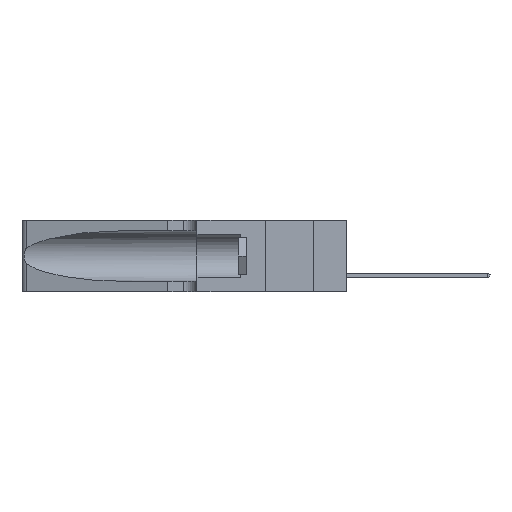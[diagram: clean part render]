
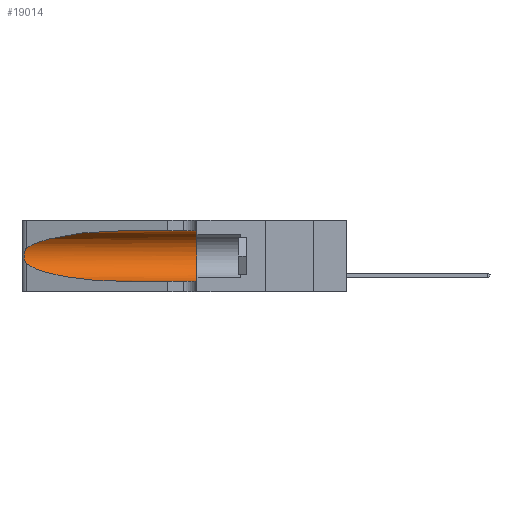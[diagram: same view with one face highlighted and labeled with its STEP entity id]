
A CAD part, left-side view. The second image highlights one B-rep face of the part: STEP entity #19014.
In plain terms, the highlighted cylindrical face has radius 3.308 mm (diameter 6.617 mm), a partial arc.
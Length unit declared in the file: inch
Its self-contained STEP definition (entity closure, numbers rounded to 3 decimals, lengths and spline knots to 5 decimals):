
#493 = VERTEX_POINT ( 'NONE', #6409 ) ;
#699 = EDGE_CURVE ( 'NONE', #23663, #19252, #7303, .T. ) ;
#864 = CARTESIAN_POINT ( 'NONE',  ( 0.1305, 0.35, 0.05475 ) ) ;
#1110 = EDGE_CURVE ( 'NONE', #493, #20791, #5302, .T. ) ;
#1565 = CARTESIAN_POINT ( 'NONE',  ( 0.26018, 1.23835, 0.19895 ) ) ;
#2272 = DIRECTION ( 'NONE',  ( 0., -1., 0. ) ) ;
#2475 = CYLINDRICAL_SURFACE ( 'NONE', #6468, 0.13025 ) ;
#3185 = DIRECTION ( 'NONE',  ( 0., 1., 0. ) ) ;
#3629 = CARTESIAN_POINT ( 'NONE',  ( 0.18966, 0.96281, 0.31525 ) ) ;
#3681 = CARTESIAN_POINT ( 'NONE',  ( 0.25856, 1.23593, 0.16098 ) ) ;
#5292 = CARTESIAN_POINT ( 'NONE',  ( 0.25487, 1.22718, 0.22369 ) ) ;
#5302 = LINE ( 'NONE', #24086, #6964 ) ;
#5741 = CARTESIAN_POINT ( 'NONE',  ( 0.25787, 1.23484, 0.2124 ) ) ;
#6034 = CARTESIAN_POINT ( 'NONE',  ( 0.2373, 1.15595, 0.28018 ) ) ;
#6409 = CARTESIAN_POINT ( 'NONE',  ( 0.1305, 0.72297, 0.05475 ) ) ;
#6468 = AXIS2_PLACEMENT_3D ( 'NONE', #24821, #9857, #7535 ) ;
#6730 = ORIENTED_EDGE ( 'NONE', *, *, #699, .F. ) ;
#6964 = VECTOR ( 'NONE', #2272, 39.37008 ) ;
#7047 = ORIENTED_EDGE ( 'NONE', *, *, #1110, .T. ) ;
#7303 = LINE ( 'NONE', #17247, #10281 ) ;
#7535 = DIRECTION ( 'NONE',  ( 0., 0., -1. ) ) ;
#7867 = CARTESIAN_POINT ( 'NONE',  ( 0.25639, 1.23186, 0.15144 ) ) ;
#8730 = DIRECTION ( 'NONE',  ( 0., -1., 0. ) ) ;
#9497 = CARTESIAN_POINT ( 'NONE',  ( 0.1305, 0.35, 0.185 ) ) ;
#9857 = DIRECTION ( 'NONE',  ( 0., -1., 0. ) ) ;
#10097 = FACE_OUTER_BOUND ( 'NONE', #18028, .T. ) ;
#10281 = VECTOR ( 'NONE', #8730, 39.37008 ) ;
#11514 = DIRECTION ( 'NONE',  ( 0., 0., 1. ) ) ;
#11858 = CARTESIAN_POINT ( 'NONE',  ( 0.25639, 1.23184, 0.21858 ) ) ;
#12005 = CARTESIAN_POINT ( 'NONE',  ( 0.1305, 0.72297, 0.05475 ) ) ;
#12075 = AXIS2_PLACEMENT_3D ( 'NONE', #9497, #3185, #11514 ) ;
#12823 = B_SPLINE_CURVE_WITH_KNOTS ( 'NONE', 3,
 ( #18354, #22823, #11858, #5741, #24591, #1565, #16399, #20304, #26755, #3681, #20674, #7867, #16484, #24966 ),
 .UNSPECIFIED., .F., .F.,
 ( 4, 2, 2, 2, 2, 2, 4 ),
 ( 0., 0.00027, 0.00053, 0.00107, 0.0016, 0.00187, 0.00214 ),
 .UNSPECIFIED. ) ;
#13263 = ORIENTED_EDGE ( 'NONE', *, *, #19708, .T. ) ;
#13898 = CARTESIAN_POINT ( 'NONE',  ( 0.25487, 1.22718, 0.14631 ) ) ;
#14076 = CARTESIAN_POINT ( 'NONE',  ( 0.18966, 0.96281, 0.05475 ) ) ;
#14173 = CARTESIAN_POINT ( 'NONE',  ( 0.25487, 1.22718, 0.14631 ) ) ;
#14568 = EDGE_CURVE ( 'NONE', #23663, #24562, #19451, .T. ) ;
#15636 = EDGE_CURVE ( 'NONE', #24767, #493, #25606, .T. ) ;
#15726 = ORIENTED_EDGE ( 'NONE', *, *, #15636, .T. ) ;
#16330 = CARTESIAN_POINT ( 'NONE',  ( 0.1305, 0.72297, 0.31525 ) ) ;
#16399 = CARTESIAN_POINT ( 'NONE',  ( 0.26075, 1.23896, 0.19203 ) ) ;
#16484 = CARTESIAN_POINT ( 'NONE',  ( 0.25555, 1.22993, 0.14849 ) ) ;
#17247 = CARTESIAN_POINT ( 'NONE',  ( 0.1305, 1.61858, 0.31525 ) ) ;
#18028 = EDGE_LOOP ( 'NONE', ( #22558, #13263, #15726, #7047, #26158, #6730 ) ) ;
#18354 = CARTESIAN_POINT ( 'NONE',  ( 0.25487, 1.22718, 0.22369 ) ) ;
#19014 = ADVANCED_FACE ( 'NONE', ( #10097 ), #2475, .F. ) ;
#19252 = VERTEX_POINT ( 'NONE', #21077 ) ;
#19451 =( BOUNDED_CURVE ( )  B_SPLINE_CURVE ( 3, ( #16330, #3629, #6034, #27057 ),
 .UNSPECIFIED., .F., .F. ) 
 B_SPLINE_CURVE_WITH_KNOTS ( ( 4, 4 ),
 ( 1.5708, 2.84003 ),
 .UNSPECIFIED. ) 
 CURVE ( )  GEOMETRIC_REPRESENTATION_ITEM ( )  RATIONAL_B_SPLINE_CURVE ( ( 1., 0.87, 0.87, 1. ) ) 
 REPRESENTATION_ITEM ( '' )  );
#19708 = EDGE_CURVE ( 'NONE', #24562, #24767, #12823, .T. ) ;
#20304 = CARTESIAN_POINT ( 'NONE',  ( 0.26075, 1.23896, 0.178 ) ) ;
#20674 = CARTESIAN_POINT ( 'NONE',  ( 0.25789, 1.23486, 0.15765 ) ) ;
#20791 = VERTEX_POINT ( 'NONE', #864 ) ;
#21077 = CARTESIAN_POINT ( 'NONE',  ( 0.1305, 0.35, 0.31525 ) ) ;
#22142 = CIRCLE ( 'NONE', #12075, 0.13025 ) ;
#22558 = ORIENTED_EDGE ( 'NONE', *, *, #14568, .T. ) ;
#22823 = CARTESIAN_POINT ( 'NONE',  ( 0.25555, 1.22994, 0.2215 ) ) ;
#22966 = CARTESIAN_POINT ( 'NONE',  ( 0.1305, 0.72297, 0.31525 ) ) ;
#23663 = VERTEX_POINT ( 'NONE', #22966 ) ;
#24086 = CARTESIAN_POINT ( 'NONE',  ( 0.1305, 1.61858, 0.05475 ) ) ;
#24562 = VERTEX_POINT ( 'NONE', #5292 ) ;
#24591 = CARTESIAN_POINT ( 'NONE',  ( 0.25854, 1.2359, 0.20912 ) ) ;
#24767 = VERTEX_POINT ( 'NONE', #13898 ) ;
#24821 = CARTESIAN_POINT ( 'NONE',  ( 0.1305, 1.61858, 0.185 ) ) ;
#24938 = CARTESIAN_POINT ( 'NONE',  ( 0.2373, 1.15595, 0.08982 ) ) ;
#24966 = CARTESIAN_POINT ( 'NONE',  ( 0.25487, 1.22718, 0.14631 ) ) ;
#25041 = EDGE_CURVE ( 'NONE', #19252, #20791, #22142, .T. ) ;
#25606 =( BOUNDED_CURVE ( )  B_SPLINE_CURVE ( 3, ( #14173, #24938, #14076, #12005 ),
 .UNSPECIFIED., .F., .F. ) 
 B_SPLINE_CURVE_WITH_KNOTS ( ( 4, 4 ),
 ( 3.44316, 4.71239 ),
 .UNSPECIFIED. ) 
 CURVE ( )  GEOMETRIC_REPRESENTATION_ITEM ( )  RATIONAL_B_SPLINE_CURVE ( ( 1., 0.87, 0.87, 1. ) ) 
 REPRESENTATION_ITEM ( '' )  );
#26158 = ORIENTED_EDGE ( 'NONE', *, *, #25041, .F. ) ;
#26755 = CARTESIAN_POINT ( 'NONE',  ( 0.26017, 1.23833, 0.17102 ) ) ;
#27057 = CARTESIAN_POINT ( 'NONE',  ( 0.25487, 1.22718, 0.22369 ) ) ;
